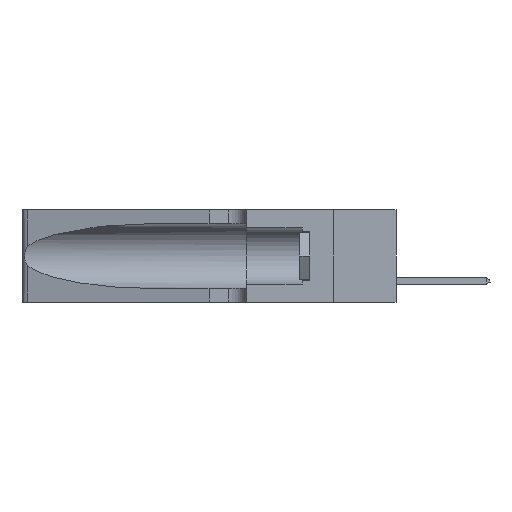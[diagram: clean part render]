
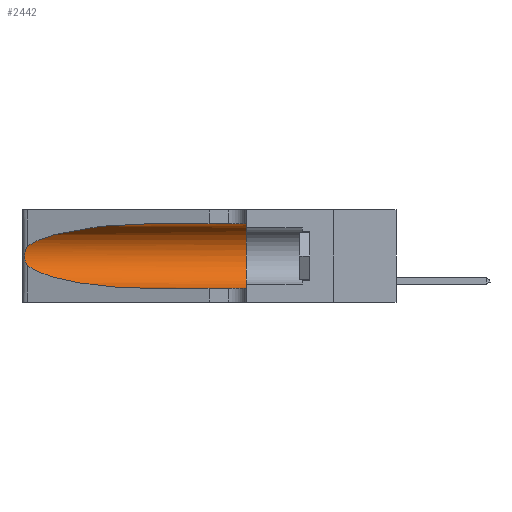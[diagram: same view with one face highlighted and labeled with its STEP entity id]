
A CAD part, left-side view. The second image highlights one B-rep face of the part: STEP entity #2442.
In plain terms, the highlighted cylindrical face has radius 3.308 mm (diameter 6.617 mm), a partial arc.
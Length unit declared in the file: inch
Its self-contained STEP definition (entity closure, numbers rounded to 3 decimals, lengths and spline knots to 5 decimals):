
#420 = CARTESIAN_POINT ( 'NONE',  ( 0.2373, 1.15595, 0.28018 ) ) ;
#617 = DIRECTION ( 'NONE',  ( 0., -1., 0. ) ) ;
#1319 = CIRCLE ( 'NONE', #29884, 0.13025 ) ;
#2036 = CARTESIAN_POINT ( 'NONE',  ( 0.25789, 1.23486, 0.15765 ) ) ;
#2442 = ADVANCED_FACE ( 'NONE', ( #30836 ), #30087, .F. ) ;
#2492 = CARTESIAN_POINT ( 'NONE',  ( 0.25487, 1.22718, 0.14631 ) ) ;
#2559 = ORIENTED_EDGE ( 'NONE', *, *, #21524, .F. ) ;
#3903 = DIRECTION ( 'NONE',  ( 0., 1., 0. ) ) ;
#4128 = LINE ( 'NONE', #10940, #31734 ) ;
#6276 = CARTESIAN_POINT ( 'NONE',  ( 0.25487, 1.22718, 0.22369 ) ) ;
#6722 = ORIENTED_EDGE ( 'NONE', *, *, #32613, .T. ) ;
#6934 = ORIENTED_EDGE ( 'NONE', *, *, #25841, .T. ) ;
#7119 = CARTESIAN_POINT ( 'NONE',  ( 0.1305, 1.61858, 0.185 ) ) ;
#7179 = CARTESIAN_POINT ( 'NONE',  ( 0.26075, 1.23896, 0.178 ) ) ;
#7391 = CARTESIAN_POINT ( 'NONE',  ( 0.25639, 1.23186, 0.15144 ) ) ;
#7725 = ORIENTED_EDGE ( 'NONE', *, *, #21429, .F. ) ;
#8334 = B_SPLINE_CURVE_WITH_KNOTS ( 'NONE', 3,
 ( #20164, #12577, #14921, #32727, #17695, #19937, #17383, #7179, #30360, #20371, #2036, #7391, #33056, #15206 ),
 .UNSPECIFIED., .F., .F.,
 ( 4, 2, 2, 2, 2, 2, 4 ),
 ( 0., 0.00027, 0.00053, 0.00107, 0.0016, 0.00187, 0.00214 ),
 .UNSPECIFIED. ) ;
#8765 = CARTESIAN_POINT ( 'NONE',  ( 0.1305, 0.72297, 0.05475 ) ) ;
#8796 = CARTESIAN_POINT ( 'NONE',  ( 0.1305, 0.35, 0.185 ) ) ;
#9176 = VERTEX_POINT ( 'NONE', #31931 ) ;
#9472 = EDGE_CURVE ( 'NONE', #15394, #24146, #12897, .T. ) ;
#10436 = CARTESIAN_POINT ( 'NONE',  ( 0.2373, 1.15595, 0.08982 ) ) ;
#10647 = CARTESIAN_POINT ( 'NONE',  ( 0.18966, 0.96281, 0.31525 ) ) ;
#10940 = CARTESIAN_POINT ( 'NONE',  ( 0.1305, 1.61858, 0.31525 ) ) ;
#11605 = VERTEX_POINT ( 'NONE', #24915 ) ;
#12485 = CARTESIAN_POINT ( 'NONE',  ( 0.1305, 0.72297, 0.05475 ) ) ;
#12577 = CARTESIAN_POINT ( 'NONE',  ( 0.25555, 1.22994, 0.2215 ) ) ;
#12897 =( BOUNDED_CURVE ( )  B_SPLINE_CURVE ( 3, ( #2492, #10436, #25438, #12485 ),
 .UNSPECIFIED., .F., .T. ) 
 B_SPLINE_CURVE_WITH_KNOTS ( ( 4, 4 ),
 ( 3.44316, 4.71239 ),
 .UNSPECIFIED. ) 
 CURVE ( )  GEOMETRIC_REPRESENTATION_ITEM ( )  RATIONAL_B_SPLINE_CURVE ( ( 1., 0.87, 0.87, 1. ) ) 
 REPRESENTATION_ITEM ( '' )  );
#14782 = ORIENTED_EDGE ( 'NONE', *, *, #9472, .T. ) ;
#14848 = DIRECTION ( 'NONE',  ( 0., 0., -1. ) ) ;
#14921 = CARTESIAN_POINT ( 'NONE',  ( 0.25639, 1.23184, 0.21858 ) ) ;
#15206 = CARTESIAN_POINT ( 'NONE',  ( 0.25487, 1.22718, 0.14631 ) ) ;
#15394 = VERTEX_POINT ( 'NONE', #22563 ) ;
#16364 =( BOUNDED_CURVE ( )  B_SPLINE_CURVE ( 3, ( #25957, #10647, #420, #6276 ),
 .UNSPECIFIED., .F., .F. ) 
 B_SPLINE_CURVE_WITH_KNOTS ( ( 4, 4 ),
 ( 1.5708, 2.84003 ),
 .UNSPECIFIED. ) 
 CURVE ( )  GEOMETRIC_REPRESENTATION_ITEM ( )  RATIONAL_B_SPLINE_CURVE ( ( 1., 0.87, 0.87, 1. ) ) 
 REPRESENTATION_ITEM ( '' )  );
#16720 = CARTESIAN_POINT ( 'NONE',  ( 0.1305, 1.61858, 0.05475 ) ) ;
#17383 = CARTESIAN_POINT ( 'NONE',  ( 0.26075, 1.23896, 0.19203 ) ) ;
#17415 = VECTOR ( 'NONE', #22811, 39.37008 ) ;
#17695 = CARTESIAN_POINT ( 'NONE',  ( 0.25854, 1.2359, 0.20912 ) ) ;
#19937 = CARTESIAN_POINT ( 'NONE',  ( 0.26018, 1.23835, 0.19895 ) ) ;
#20164 = CARTESIAN_POINT ( 'NONE',  ( 0.25487, 1.22718, 0.22369 ) ) ;
#20371 = CARTESIAN_POINT ( 'NONE',  ( 0.25856, 1.23593, 0.16098 ) ) ;
#21020 = EDGE_LOOP ( 'NONE', ( #32115, #6722, #14782, #6934, #2559, #7725 ) ) ;
#21429 = EDGE_CURVE ( 'NONE', #9176, #11605, #4128, .T. ) ;
#21524 = EDGE_CURVE ( 'NONE', #11605, #30974, #1319, .T. ) ;
#22563 = CARTESIAN_POINT ( 'NONE',  ( 0.25487, 1.22718, 0.14631 ) ) ;
#22811 = DIRECTION ( 'NONE',  ( 0., -1., 0. ) ) ;
#23838 = EDGE_CURVE ( 'NONE', #9176, #24030, #16364, .T. ) ;
#24030 = VERTEX_POINT ( 'NONE', #31589 ) ;
#24146 = VERTEX_POINT ( 'NONE', #8765 ) ;
#24915 = CARTESIAN_POINT ( 'NONE',  ( 0.1305, 0.35, 0.31525 ) ) ;
#25046 = DIRECTION ( 'NONE',  ( 0., 0., 1. ) ) ;
#25396 = LINE ( 'NONE', #16720, #17415 ) ;
#25438 = CARTESIAN_POINT ( 'NONE',  ( 0.18966, 0.96281, 0.05475 ) ) ;
#25841 = EDGE_CURVE ( 'NONE', #24146, #30974, #25396, .T. ) ;
#25957 = CARTESIAN_POINT ( 'NONE',  ( 0.1305, 0.72297, 0.31525 ) ) ;
#25958 = CARTESIAN_POINT ( 'NONE',  ( 0.1305, 0.35, 0.05475 ) ) ;
#26544 = AXIS2_PLACEMENT_3D ( 'NONE', #7119, #30180, #14848 ) ;
#29884 = AXIS2_PLACEMENT_3D ( 'NONE', #8796, #3903, #25046 ) ;
#30087 = CYLINDRICAL_SURFACE ( 'NONE', #26544, 0.13025 ) ;
#30180 = DIRECTION ( 'NONE',  ( 0., -1., 0. ) ) ;
#30360 = CARTESIAN_POINT ( 'NONE',  ( 0.26017, 1.23833, 0.17102 ) ) ;
#30836 = FACE_OUTER_BOUND ( 'NONE', #21020, .T. ) ;
#30974 = VERTEX_POINT ( 'NONE', #25958 ) ;
#31589 = CARTESIAN_POINT ( 'NONE',  ( 0.25487, 1.22718, 0.22369 ) ) ;
#31734 = VECTOR ( 'NONE', #617, 39.37008 ) ;
#31931 = CARTESIAN_POINT ( 'NONE',  ( 0.1305, 0.72297, 0.31525 ) ) ;
#32115 = ORIENTED_EDGE ( 'NONE', *, *, #23838, .T. ) ;
#32613 = EDGE_CURVE ( 'NONE', #24030, #15394, #8334, .T. ) ;
#32727 = CARTESIAN_POINT ( 'NONE',  ( 0.25787, 1.23484, 0.2124 ) ) ;
#33056 = CARTESIAN_POINT ( 'NONE',  ( 0.25555, 1.22993, 0.14849 ) ) ;
